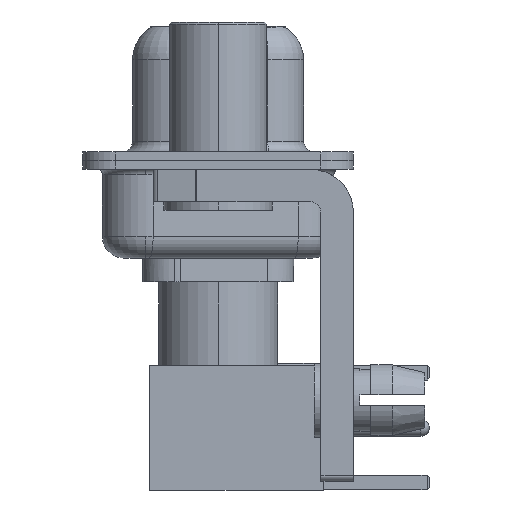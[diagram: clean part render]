
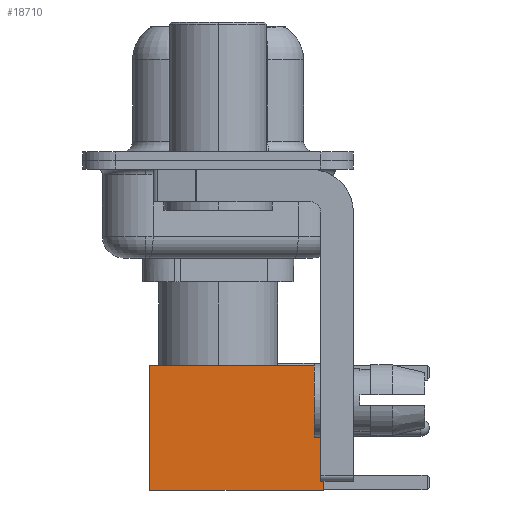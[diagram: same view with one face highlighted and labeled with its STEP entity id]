
A CAD part, left-side view. The second image highlights one B-rep face of the part: STEP entity #18710.
In plain terms, the highlighted face is planar.
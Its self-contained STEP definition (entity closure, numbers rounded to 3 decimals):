
#855 = AXIS2_PLACEMENT_3D ( 'NONE', #7522, #3677, #9451 ) ;
#1058 = LINE ( 'NONE', #18655, #19374 ) ;
#3677 = DIRECTION ( 'NONE',  ( 0., 1., 0. ) ) ;
#4438 = DIRECTION ( 'NONE',  ( -1., 0., 0. ) ) ;
#4905 = CARTESIAN_POINT ( 'NONE',  ( -2.875, 2.875, 0. ) ) ;
#6267 = VERTEX_POINT ( 'NONE', #8998 ) ;
#6824 = DIRECTION ( 'NONE',  ( 0., 0., -1. ) ) ;
#6952 = LINE ( 'NONE', #16851, #15691 ) ;
#7201 = DIRECTION ( 'NONE',  ( 0., 0., -1. ) ) ;
#7522 = CARTESIAN_POINT ( 'NONE',  ( 2.875, 2.875, 0. ) ) ;
#8158 = CARTESIAN_POINT ( 'NONE',  ( 0., 2.875, 8. ) ) ;
#8998 = CARTESIAN_POINT ( 'NONE',  ( 2.875, 2.875, 0. ) ) ;
#9451 = DIRECTION ( 'NONE',  ( 0., 0., 1. ) ) ;
#9859 = CARTESIAN_POINT ( 'NONE',  ( 2.875, 2.875, 8. ) ) ;
#10923 = CARTESIAN_POINT ( 'NONE',  ( 0., 2.875, 0. ) ) ;
#11483 = VECTOR ( 'NONE', #4438, 1000. ) ;
#13308 = FACE_OUTER_BOUND ( 'NONE', #22210, .T. ) ;
#13454 = VERTEX_POINT ( 'NONE', #16934 ) ;
#14186 = VERTEX_POINT ( 'NONE', #4905 ) ;
#14802 = VECTOR ( 'NONE', #22502, 1000. ) ;
#14991 = PLANE ( 'NONE',  #855 ) ;
#15691 = VECTOR ( 'NONE', #6824, 1000. ) ;
#15914 = ORIENTED_EDGE ( 'NONE', *, *, #20978, .T. ) ;
#16601 = LINE ( 'NONE', #10923, #14802 ) ;
#16851 = CARTESIAN_POINT ( 'NONE',  ( -2.875, 2.875, 0. ) ) ;
#16934 = CARTESIAN_POINT ( 'NONE',  ( -2.875, 2.875, 8. ) ) ;
#17919 = LINE ( 'NONE', #8158, #11483 ) ;
#18655 = CARTESIAN_POINT ( 'NONE',  ( 2.875, 2.875, 0. ) ) ;
#18710 = ADVANCED_FACE ( 'NONE', ( #13308 ), #14991, .T. ) ;
#18919 = EDGE_CURVE ( 'NONE', #23223, #13454, #17919, .T. ) ;
#19374 = VECTOR ( 'NONE', #7201, 1000. ) ;
#20978 = EDGE_CURVE ( 'NONE', #6267, #14186, #16601, .T. ) ;
#21486 = ORIENTED_EDGE ( 'NONE', *, *, #18919, .F. ) ;
#22117 = ORIENTED_EDGE ( 'NONE', *, *, #22358, .F. ) ;
#22210 = EDGE_LOOP ( 'NONE', ( #24861, #15914, #22117, #21486 ) ) ;
#22358 = EDGE_CURVE ( 'NONE', #13454, #14186, #6952, .T. ) ;
#22368 = EDGE_CURVE ( 'NONE', #23223, #6267, #1058, .T. ) ;
#22502 = DIRECTION ( 'NONE',  ( -1., 0., 0. ) ) ;
#23223 = VERTEX_POINT ( 'NONE', #9859 ) ;
#24861 = ORIENTED_EDGE ( 'NONE', *, *, #22368, .T. ) ;
